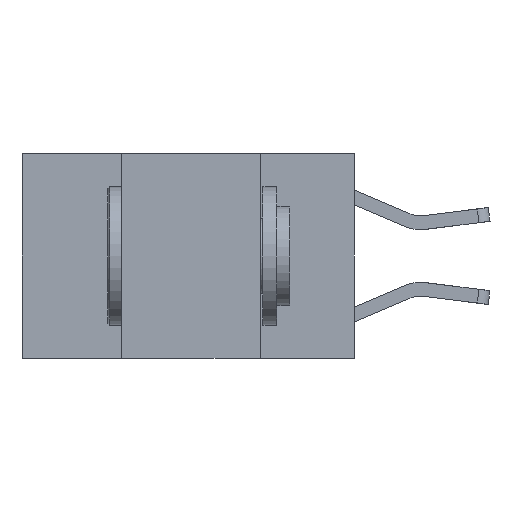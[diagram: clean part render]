
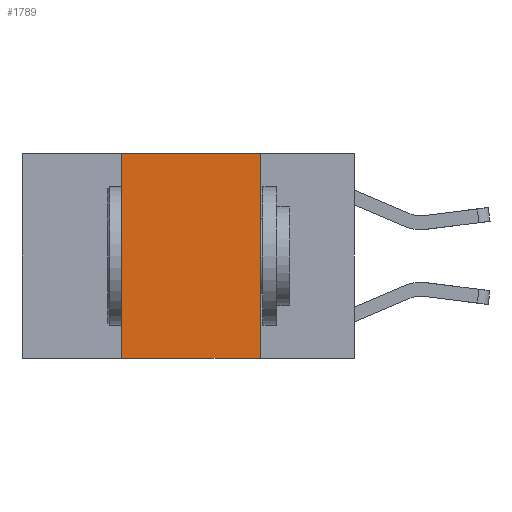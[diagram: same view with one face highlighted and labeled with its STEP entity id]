
A CAD part, left-side view. The second image highlights one B-rep face of the part: STEP entity #1789.
In plain terms, the highlighted planar face has unit normal (-1, 0, 0).
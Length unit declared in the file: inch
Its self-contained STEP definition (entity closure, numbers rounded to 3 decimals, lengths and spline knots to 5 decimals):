
#131 = LINE ( 'NONE', #8760, #396 ) ;
#290 = LINE ( 'NONE', #9713, #9504 ) ;
#396 = VECTOR ( 'NONE', #1095, 39.37008 ) ;
#450 = CARTESIAN_POINT ( 'NONE',  ( 0., 0.6, 0. ) ) ;
#460 = ORIENTED_EDGE ( 'NONE', *, *, #10921, .F. ) ;
#1095 = DIRECTION ( 'NONE',  ( 0., 0., 1. ) ) ;
#1427 = EDGE_CURVE ( 'NONE', #11179, #5174, #131, .T. ) ;
#1780 = FACE_OUTER_BOUND ( 'NONE', #8498, .T. ) ;
#1789 = ADVANCED_FACE ( 'NONE', ( #1780 ), #5250, .F. ) ;
#1950 = ORIENTED_EDGE ( 'NONE', *, *, #10644, .F. ) ;
#2242 = LINE ( 'NONE', #450, #9868 ) ;
#3105 = VERTEX_POINT ( 'NONE', #10490 ) ;
#3741 = VERTEX_POINT ( 'NONE', #9135 ) ;
#3779 = CARTESIAN_POINT ( 'NONE',  ( 0., 0.6, -0.37 ) ) ;
#3839 = VECTOR ( 'NONE', #7997, 39.37008 ) ;
#4051 = DIRECTION ( 'NONE',  ( 1., 0., 0. ) ) ;
#4455 = AXIS2_PLACEMENT_3D ( 'NONE', #8748, #4051, #7593 ) ;
#4516 = LINE ( 'NONE', #3779, #3839 ) ;
#5032 = CARTESIAN_POINT ( 'NONE',  ( 0., 0.42, 0. ) ) ;
#5174 = VERTEX_POINT ( 'NONE', #5032 ) ;
#5250 = PLANE ( 'NONE',  #4455 ) ;
#6404 = DIRECTION ( 'NONE',  ( 0., 0., -1. ) ) ;
#7484 = DIRECTION ( 'NONE',  ( 0., -1., 0. ) ) ;
#7593 = DIRECTION ( 'NONE',  ( 0., 0., -1. ) ) ;
#7778 = ORIENTED_EDGE ( 'NONE', *, *, #10507, .T. ) ;
#7797 = CARTESIAN_POINT ( 'NONE',  ( 0., 0.42, -0.37 ) ) ;
#7997 = DIRECTION ( 'NONE',  ( 0., -1., 0. ) ) ;
#8498 = EDGE_LOOP ( 'NONE', ( #460, #1950, #9299, #7778 ) ) ;
#8748 = CARTESIAN_POINT ( 'NONE',  ( 0., 0.6, 0. ) ) ;
#8760 = CARTESIAN_POINT ( 'NONE',  ( 0., 0.42, 0. ) ) ;
#9135 = CARTESIAN_POINT ( 'NONE',  ( 0., 0.17, 0. ) ) ;
#9299 = ORIENTED_EDGE ( 'NONE', *, *, #1427, .F. ) ;
#9504 = VECTOR ( 'NONE', #6404, 39.37008 ) ;
#9713 = CARTESIAN_POINT ( 'NONE',  ( 0., 0.17, 0. ) ) ;
#9868 = VECTOR ( 'NONE', #7484, 39.37008 ) ;
#10490 = CARTESIAN_POINT ( 'NONE',  ( 0., 0.17, -0.37 ) ) ;
#10507 = EDGE_CURVE ( 'NONE', #11179, #3105, #4516, .T. ) ;
#10644 = EDGE_CURVE ( 'NONE', #5174, #3741, #2242, .T. ) ;
#10921 = EDGE_CURVE ( 'NONE', #3741, #3105, #290, .T. ) ;
#11179 = VERTEX_POINT ( 'NONE', #7797 ) ;
